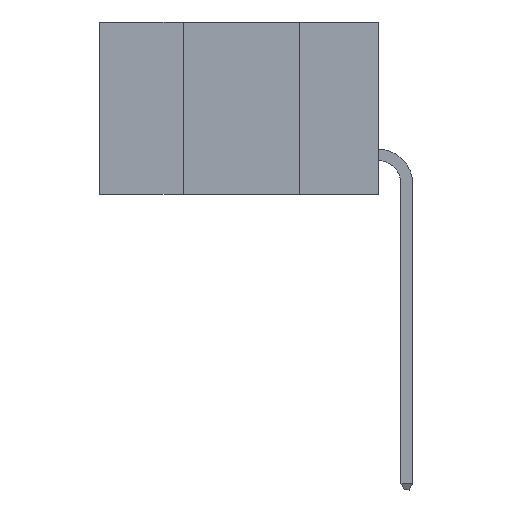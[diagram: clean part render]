
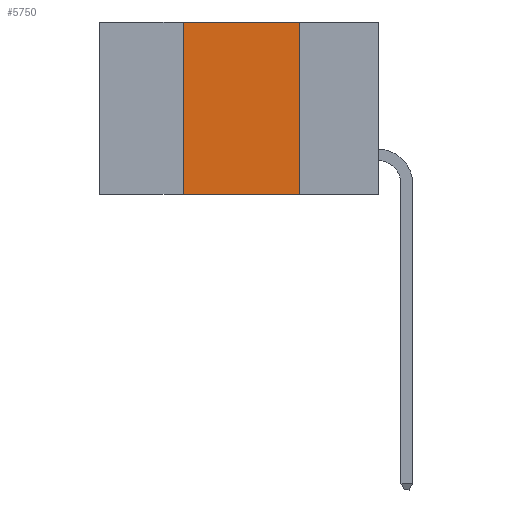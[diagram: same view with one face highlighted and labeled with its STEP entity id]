
A CAD part, left-side view. The second image highlights one B-rep face of the part: STEP entity #5750.
In plain terms, the highlighted planar face has unit normal (-1, 0, 0).
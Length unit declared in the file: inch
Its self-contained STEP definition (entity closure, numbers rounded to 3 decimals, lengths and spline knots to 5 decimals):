
#155 = CARTESIAN_POINT ( 'NONE',  ( 0., 0.42, -0.37 ) ) ;
#228 = VECTOR ( 'NONE', #4709, 39.37008 ) ;
#2028 = CARTESIAN_POINT ( 'NONE',  ( 0., 0.17, 0. ) ) ;
#2257 = CARTESIAN_POINT ( 'NONE',  ( 0., 0.17, 0. ) ) ;
#2613 = PLANE ( 'NONE',  #4903 ) ;
#2776 = EDGE_CURVE ( 'NONE', #9757, #5684, #9083, .T. ) ;
#2914 = EDGE_CURVE ( 'NONE', #4833, #9757, #9648, .T. ) ;
#2976 = ORIENTED_EDGE ( 'NONE', *, *, #8525, .T. ) ;
#3532 = EDGE_LOOP ( 'NONE', ( #5159, #10401, #4659, #2976 ) ) ;
#3956 = CARTESIAN_POINT ( 'NONE',  ( 0., 0.6, -0.37 ) ) ;
#4451 = DIRECTION ( 'NONE',  ( 0., 0., -1. ) ) ;
#4469 = CARTESIAN_POINT ( 'NONE',  ( 0., 0.6, 0. ) ) ;
#4496 = VERTEX_POINT ( 'NONE', #155 ) ;
#4575 = DIRECTION ( 'NONE',  ( 1., 0., 0. ) ) ;
#4659 = ORIENTED_EDGE ( 'NONE', *, *, #6807, .F. ) ;
#4709 = DIRECTION ( 'NONE',  ( 0., 0., -1. ) ) ;
#4833 = VERTEX_POINT ( 'NONE', #5315 ) ;
#4903 = AXIS2_PLACEMENT_3D ( 'NONE', #6796, #4575, #4451 ) ;
#5159 = ORIENTED_EDGE ( 'NONE', *, *, #2776, .F. ) ;
#5315 = CARTESIAN_POINT ( 'NONE',  ( 0., 0.42, 0. ) ) ;
#5684 = VERTEX_POINT ( 'NONE', #7671 ) ;
#5742 = CARTESIAN_POINT ( 'NONE',  ( 0., 0.42, 0. ) ) ;
#5750 = ADVANCED_FACE ( 'NONE', ( #5969 ), #2613, .F. ) ;
#5969 = FACE_OUTER_BOUND ( 'NONE', #3532, .T. ) ;
#6526 = LINE ( 'NONE', #5742, #8802 ) ;
#6769 = DIRECTION ( 'NONE',  ( 0., -1., 0. ) ) ;
#6796 = CARTESIAN_POINT ( 'NONE',  ( 0., 0.6, 0. ) ) ;
#6807 = EDGE_CURVE ( 'NONE', #4496, #4833, #6526, .T. ) ;
#7334 = VECTOR ( 'NONE', #10202, 39.37008 ) ;
#7648 = VECTOR ( 'NONE', #6769, 39.37008 ) ;
#7671 = CARTESIAN_POINT ( 'NONE',  ( 0., 0.17, -0.37 ) ) ;
#8525 = EDGE_CURVE ( 'NONE', #4496, #5684, #9340, .T. ) ;
#8802 = VECTOR ( 'NONE', #9004, 39.37008 ) ;
#9004 = DIRECTION ( 'NONE',  ( 0., 0., 1. ) ) ;
#9083 = LINE ( 'NONE', #2257, #228 ) ;
#9340 = LINE ( 'NONE', #3956, #7334 ) ;
#9648 = LINE ( 'NONE', #4469, #7648 ) ;
#9757 = VERTEX_POINT ( 'NONE', #2028 ) ;
#10202 = DIRECTION ( 'NONE',  ( 0., -1., 0. ) ) ;
#10401 = ORIENTED_EDGE ( 'NONE', *, *, #2914, .F. ) ;
